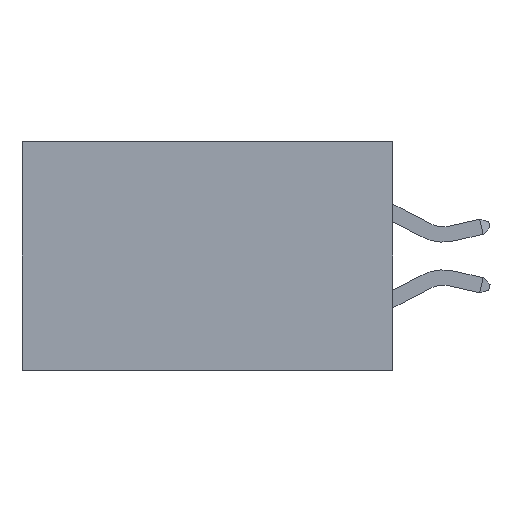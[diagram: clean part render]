
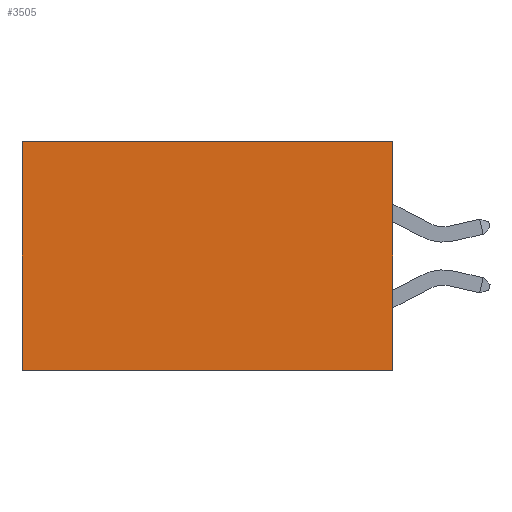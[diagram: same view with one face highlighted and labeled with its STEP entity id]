
A CAD part, left-side view. The second image highlights one B-rep face of the part: STEP entity #3505.
In plain terms, the highlighted planar face has unit normal (-1, 0, 0).
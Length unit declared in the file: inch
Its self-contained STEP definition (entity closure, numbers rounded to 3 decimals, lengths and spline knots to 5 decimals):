
#1065 = LINE ( 'NONE', #5555, #4865 ) ;
#2046 = EDGE_CURVE ( 'NONE', #14487, #7871, #1065, .T. ) ;
#2526 = ORIENTED_EDGE ( 'NONE', *, *, #2046, .F. ) ;
#2864 = CARTESIAN_POINT ( 'NONE',  ( 0.2875, 0., 0. ) ) ;
#3505 = ADVANCED_FACE ( 'NONE', ( #23105 ), #16193, .F. ) ;
#3848 = LINE ( 'NONE', #4124, #18002 ) ;
#4124 = CARTESIAN_POINT ( 'NONE',  ( 0.2875, 0., -0.37 ) ) ;
#4626 = EDGE_CURVE ( 'NONE', #14487, #13899, #11224, .T. ) ;
#4865 = VECTOR ( 'NONE', #15215, 39.37008 ) ;
#4899 = CARTESIAN_POINT ( 'NONE',  ( 0.2875, 0., 0. ) ) ;
#4979 = DIRECTION ( 'NONE',  ( 1., 0., 0. ) ) ;
#5555 = CARTESIAN_POINT ( 'NONE',  ( 0.2875, 0., 0. ) ) ;
#6698 = DIRECTION ( 'NONE',  ( 0., 1., 0. ) ) ;
#6927 = DIRECTION ( 'NONE',  ( 0., 0., -1. ) ) ;
#6951 = VERTEX_POINT ( 'NONE', #12235 ) ;
#6958 = CARTESIAN_POINT ( 'NONE',  ( 0.2875, 0.6, 0. ) ) ;
#7871 = VERTEX_POINT ( 'NONE', #17707 ) ;
#8834 = VECTOR ( 'NONE', #19439, 39.37008 ) ;
#10562 = CARTESIAN_POINT ( 'NONE',  ( 0.2875, 0., 0. ) ) ;
#10844 = EDGE_LOOP ( 'NONE', ( #15367, #23870, #2526, #24234 ) ) ;
#11224 = LINE ( 'NONE', #4899, #12405 ) ;
#11715 = DIRECTION ( 'NONE',  ( 0., 1., 0. ) ) ;
#12002 = CARTESIAN_POINT ( 'NONE',  ( 0.2875, 0.6, 0. ) ) ;
#12235 = CARTESIAN_POINT ( 'NONE',  ( 0.2875, 0.6, -0.37 ) ) ;
#12405 = VECTOR ( 'NONE', #6698, 39.37008 ) ;
#13899 = VERTEX_POINT ( 'NONE', #6958 ) ;
#14487 = VERTEX_POINT ( 'NONE', #2864 ) ;
#15215 = DIRECTION ( 'NONE',  ( 0., 0., -1. ) ) ;
#15367 = ORIENTED_EDGE ( 'NONE', *, *, #23814, .T. ) ;
#16028 = EDGE_CURVE ( 'NONE', #7871, #6951, #3848, .T. ) ;
#16193 = PLANE ( 'NONE',  #23885 ) ;
#17707 = CARTESIAN_POINT ( 'NONE',  ( 0.2875, 0., -0.37 ) ) ;
#18002 = VECTOR ( 'NONE', #11715, 39.37008 ) ;
#19439 = DIRECTION ( 'NONE',  ( 0., 0., -1. ) ) ;
#19487 = LINE ( 'NONE', #12002, #8834 ) ;
#23105 = FACE_OUTER_BOUND ( 'NONE', #10844, .T. ) ;
#23814 = EDGE_CURVE ( 'NONE', #13899, #6951, #19487, .T. ) ;
#23870 = ORIENTED_EDGE ( 'NONE', *, *, #16028, .F. ) ;
#23885 = AXIS2_PLACEMENT_3D ( 'NONE', #10562, #4979, #6927 ) ;
#24234 = ORIENTED_EDGE ( 'NONE', *, *, #4626, .T. ) ;
